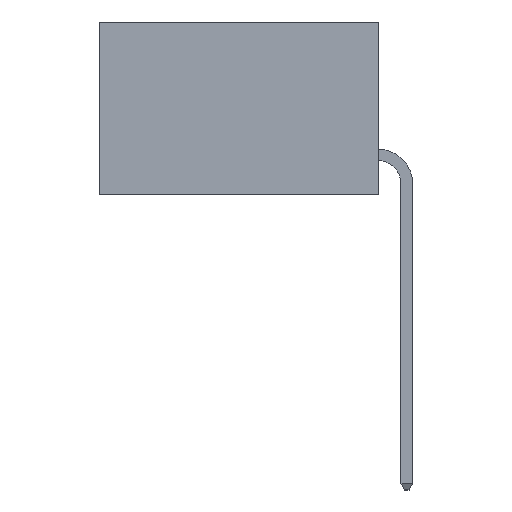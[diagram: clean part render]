
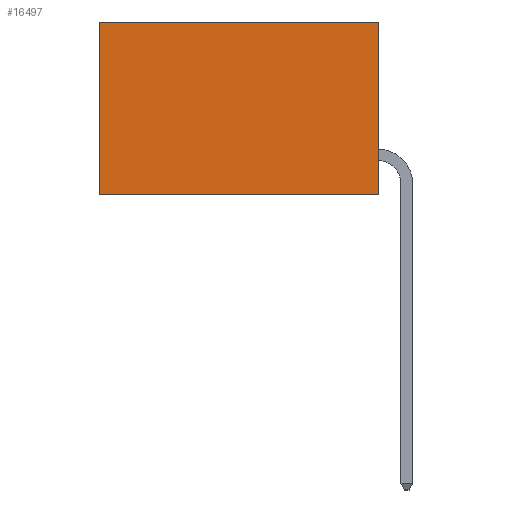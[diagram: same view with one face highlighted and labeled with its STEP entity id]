
A CAD part, left-side view. The second image highlights one B-rep face of the part: STEP entity #16497.
In plain terms, the highlighted planar face has unit normal (-1, 0, 0).
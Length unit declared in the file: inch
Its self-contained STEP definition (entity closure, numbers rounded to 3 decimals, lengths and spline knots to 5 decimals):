
#330 = PLANE ( 'NONE',  #2991 ) ;
#1371 = CARTESIAN_POINT ( 'NONE',  ( 0.2615, 0., 0. ) ) ;
#1931 = CARTESIAN_POINT ( 'NONE',  ( 0.2615, 0., -0.37 ) ) ;
#1989 = CARTESIAN_POINT ( 'NONE',  ( 0.2615, 0.6, 0. ) ) ;
#2089 = ORIENTED_EDGE ( 'NONE', *, *, #16372, .T. ) ;
#2526 = VERTEX_POINT ( 'NONE', #16436 ) ;
#2645 = DIRECTION ( 'NONE',  ( 0., 1., 0. ) ) ;
#2991 = AXIS2_PLACEMENT_3D ( 'NONE', #4264, #13352, #5605 ) ;
#3143 = EDGE_CURVE ( 'NONE', #16764, #13116, #15051, .T. ) ;
#3771 = DIRECTION ( 'NONE',  ( 0., 0., -1. ) ) ;
#4264 = CARTESIAN_POINT ( 'NONE',  ( 0.2615, 0., -0.37 ) ) ;
#4705 = ORIENTED_EDGE ( 'NONE', *, *, #15786, .T. ) ;
#4887 = CARTESIAN_POINT ( 'NONE',  ( 0.2615, 0.6, -0.37 ) ) ;
#5605 = DIRECTION ( 'NONE',  ( 0., 0., -1. ) ) ;
#6197 = DIRECTION ( 'NONE',  ( 0., 0., -1. ) ) ;
#6212 = FACE_OUTER_BOUND ( 'NONE', #12014, .T. ) ;
#6344 = ORIENTED_EDGE ( 'NONE', *, *, #3143, .F. ) ;
#6581 = ORIENTED_EDGE ( 'NONE', *, *, #14399, .F. ) ;
#6999 = CARTESIAN_POINT ( 'NONE',  ( 0.2615, 0., -0.37 ) ) ;
#7064 = DIRECTION ( 'NONE',  ( 0., 1., 0. ) ) ;
#8688 = LINE ( 'NONE', #1371, #15165 ) ;
#8984 = VERTEX_POINT ( 'NONE', #1989 ) ;
#11132 = LINE ( 'NONE', #4887, #14988 ) ;
#11987 = VECTOR ( 'NONE', #3771, 39.37008 ) ;
#12014 = EDGE_LOOP ( 'NONE', ( #4705, #6581, #6344, #2089 ) ) ;
#12376 = VECTOR ( 'NONE', #7064, 39.37008 ) ;
#12618 = CARTESIAN_POINT ( 'NONE',  ( 0.2615, 0., 0. ) ) ;
#12783 = LINE ( 'NONE', #16151, #12376 ) ;
#13116 = VERTEX_POINT ( 'NONE', #6999 ) ;
#13352 = DIRECTION ( 'NONE',  ( 1., 0., 0. ) ) ;
#14399 = EDGE_CURVE ( 'NONE', #13116, #2526, #12783, .T. ) ;
#14988 = VECTOR ( 'NONE', #6197, 39.37008 ) ;
#15051 = LINE ( 'NONE', #1931, #11987 ) ;
#15165 = VECTOR ( 'NONE', #2645, 39.37008 ) ;
#15786 = EDGE_CURVE ( 'NONE', #8984, #2526, #11132, .T. ) ;
#16151 = CARTESIAN_POINT ( 'NONE',  ( 0.2615, 0., -0.37 ) ) ;
#16372 = EDGE_CURVE ( 'NONE', #16764, #8984, #8688, .T. ) ;
#16436 = CARTESIAN_POINT ( 'NONE',  ( 0.2615, 0.6, -0.37 ) ) ;
#16497 = ADVANCED_FACE ( 'NONE', ( #6212 ), #330, .F. ) ;
#16764 = VERTEX_POINT ( 'NONE', #12618 ) ;
